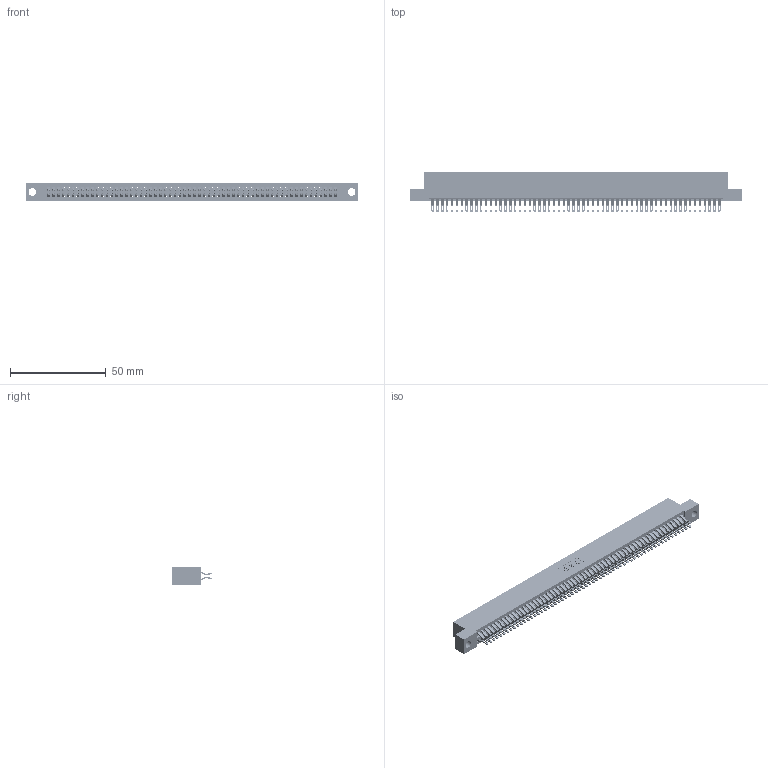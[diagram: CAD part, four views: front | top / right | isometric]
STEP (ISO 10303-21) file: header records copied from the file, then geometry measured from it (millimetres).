
FILE_DESCRIPTION (( 'STEP AP203' ), '1' );
FILE_NAME ('345-120-555-204.STEP', '2021-05-25T17:05:58', ( '' ), ( '' ), 'SwSTEP 2.0', 'SolidWorks 2020', '' );
FILE_SCHEMA (( 'CONFIG_CONTROL_DESIGN' ));
Length unit declared in the file: inch
Products named in the file (3): 345-292-001_555 Tail; 345-120-555-204; 345 Part_Flush Mounting Lugs - 0.156 Dia-TI
Assembly tree (121 placements, depth 2):
  345-120-555-204
    345 Part_Flush Mounting Lugs - 0.156 Dia-TI
    345-292-001_555 Tail  x120
Bounding box: 173.61 x 21.13 x 9.4 mm (x, y, z)
Volume: 17273.8 mm3; surface area: 26944.3 mm2
Topology: 121 solids, 121 shells, 6860 faces, 21617 edges, 14410 vertices
Faces by surface type: plane 3814, cylinder 3046
Entity records: 45399 total; most frequent: CARTESIAN_POINT 7632, ORIENTED_EDGE 7534, DIRECTION 6675, EDGE_CURVE 3767, VECTOR 3375, LINE 3375, VERTEX_POINT 2510, AXIS2_PLACEMENT_3D 1650
